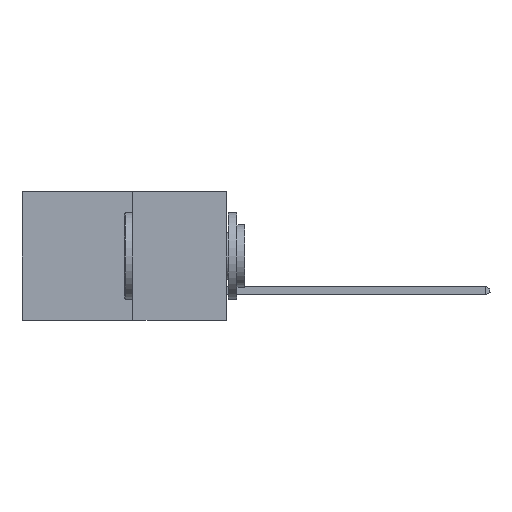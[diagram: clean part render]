
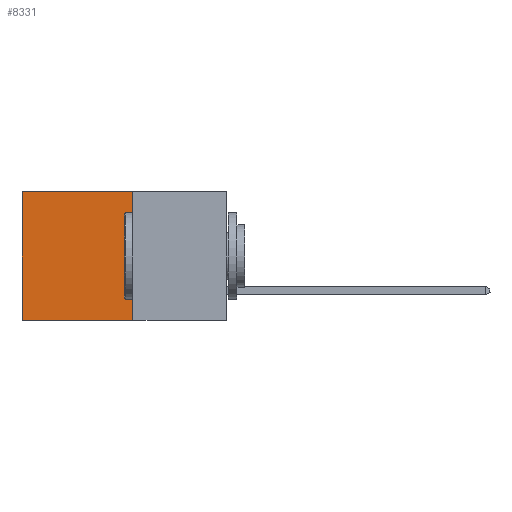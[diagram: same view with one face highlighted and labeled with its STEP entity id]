
A CAD part, left-side view. The second image highlights one B-rep face of the part: STEP entity #8331.
In plain terms, the highlighted planar face has unit normal (-1, 0, 0).
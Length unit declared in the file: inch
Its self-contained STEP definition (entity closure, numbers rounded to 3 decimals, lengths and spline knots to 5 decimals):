
#101 = ORIENTED_EDGE ( 'NONE', *, *, #5074, .F. ) ;
#531 = DIRECTION ( 'NONE',  ( 0., 0., -1. ) ) ;
#1453 = CARTESIAN_POINT ( 'NONE',  ( 0.277, 0.27, 0. ) ) ;
#1610 = ORIENTED_EDGE ( 'NONE', *, *, #6581, .T. ) ;
#1742 = DIRECTION ( 'NONE',  ( 0., 1., 0. ) ) ;
#2251 = CARTESIAN_POINT ( 'NONE',  ( 0.277, 0.27, -0.37 ) ) ;
#2423 = CARTESIAN_POINT ( 'NONE',  ( 0.277, 0.59, 0. ) ) ;
#2786 = ORIENTED_EDGE ( 'NONE', *, *, #10929, .T. ) ;
#2890 = VERTEX_POINT ( 'NONE', #2423 ) ;
#2912 = ORIENTED_EDGE ( 'NONE', *, *, #5905, .F. ) ;
#2948 = VECTOR ( 'NONE', #531, 39.37008 ) ;
#3290 = LINE ( 'NONE', #13996, #2948 ) ;
#3783 = VERTEX_POINT ( 'NONE', #6789 ) ;
#5074 = EDGE_CURVE ( 'NONE', #3783, #5089, #7015, .T. ) ;
#5089 = VERTEX_POINT ( 'NONE', #2251 ) ;
#5905 = EDGE_CURVE ( 'NONE', #5089, #12426, #9363, .T. ) ;
#6555 = LINE ( 'NONE', #1453, #9165 ) ;
#6581 = EDGE_CURVE ( 'NONE', #3783, #2890, #6555, .T. ) ;
#6789 = CARTESIAN_POINT ( 'NONE',  ( 0.277, 0.27, 0. ) ) ;
#7015 = LINE ( 'NONE', #10771, #12531 ) ;
#7323 = EDGE_LOOP ( 'NONE', ( #2786, #2912, #101, #1610 ) ) ;
#8331 = ADVANCED_FACE ( 'NONE', ( #12708 ), #10854, .F. ) ;
#9019 = VECTOR ( 'NONE', #11730, 39.37008 ) ;
#9165 = VECTOR ( 'NONE', #1742, 39.37008 ) ;
#9363 = LINE ( 'NONE', #12467, #9019 ) ;
#10662 = DIRECTION ( 'NONE',  ( 0., 0., -1. ) ) ;
#10702 = DIRECTION ( 'NONE',  ( 1., 0., 0. ) ) ;
#10771 = CARTESIAN_POINT ( 'NONE',  ( 0.277, 0.27, -0.37 ) ) ;
#10775 = DIRECTION ( 'NONE',  ( 0., 0., -1. ) ) ;
#10805 = CARTESIAN_POINT ( 'NONE',  ( 0.277, 0.27, -0.37 ) ) ;
#10854 = PLANE ( 'NONE',  #13714 ) ;
#10929 = EDGE_CURVE ( 'NONE', #2890, #12426, #3290, .T. ) ;
#11040 = CARTESIAN_POINT ( 'NONE',  ( 0.277, 0.59, -0.37 ) ) ;
#11730 = DIRECTION ( 'NONE',  ( 0., 1., 0. ) ) ;
#12426 = VERTEX_POINT ( 'NONE', #11040 ) ;
#12467 = CARTESIAN_POINT ( 'NONE',  ( 0.277, 0.27, -0.37 ) ) ;
#12531 = VECTOR ( 'NONE', #10775, 39.37008 ) ;
#12708 = FACE_OUTER_BOUND ( 'NONE', #7323, .T. ) ;
#13714 = AXIS2_PLACEMENT_3D ( 'NONE', #10805, #10702, #10662 ) ;
#13996 = CARTESIAN_POINT ( 'NONE',  ( 0.277, 0.59, -0.37 ) ) ;
